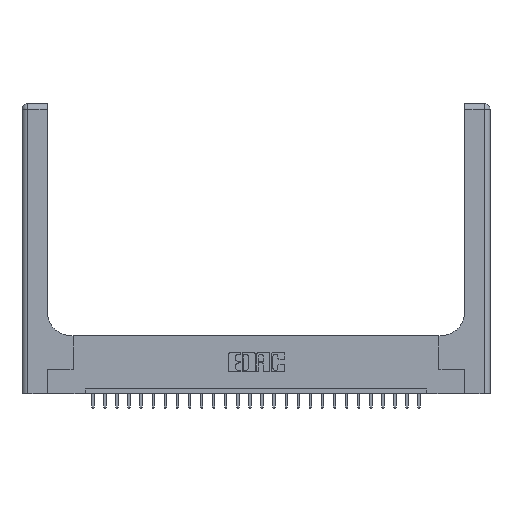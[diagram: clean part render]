
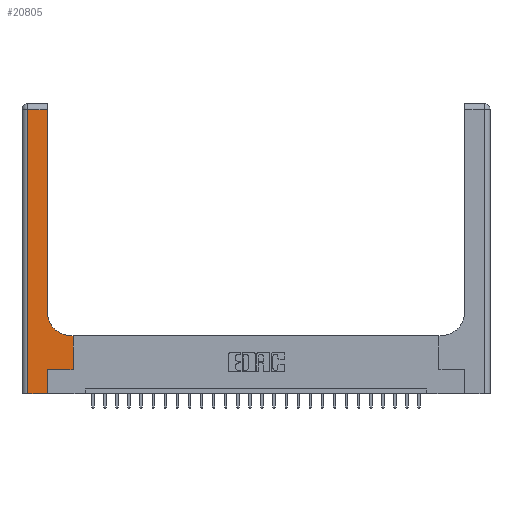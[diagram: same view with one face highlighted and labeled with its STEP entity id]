
A CAD part, top view. The second image highlights one B-rep face of the part: STEP entity #20805.
In plain terms, the highlighted planar face has unit normal (0, 0, 1).
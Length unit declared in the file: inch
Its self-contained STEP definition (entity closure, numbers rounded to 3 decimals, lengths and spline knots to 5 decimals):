
#198 = VERTEX_POINT ( 'NONE', #9054 ) ;
#216 = EDGE_CURVE ( 'NONE', #22967, #11953, #3012, .T. ) ;
#431 = CARTESIAN_POINT ( 'NONE',  ( 0.51, 0.6, 0.37 ) ) ;
#540 = ORIENTED_EDGE ( 'NONE', *, *, #24052, .T. ) ;
#685 = LINE ( 'NONE', #8869, #21875 ) ;
#1987 = CARTESIAN_POINT ( 'NONE',  ( 0.265, 0.25, 0.37 ) ) ;
#2176 = VERTEX_POINT ( 'NONE', #15925 ) ;
#2447 = DIRECTION ( 'NONE',  ( 0., 1., 0. ) ) ;
#2916 = DIRECTION ( 'NONE',  ( 1., 0., 0. ) ) ;
#3012 = LINE ( 'NONE', #6914, #24234 ) ;
#3833 = EDGE_CURVE ( 'NONE', #198, #21605, #20559, .T. ) ;
#4216 = CARTESIAN_POINT ( 'NONE',  ( 0.265, 0., 0.37 ) ) ;
#4338 = LINE ( 'NONE', #15784, #7513 ) ;
#4696 = AXIS2_PLACEMENT_3D ( 'NONE', #9134, #7483, #15160 ) ;
#4815 = CARTESIAN_POINT ( 'NONE',  ( 0.265, 0.25, 0.37 ) ) ;
#4822 = CARTESIAN_POINT ( 'NONE',  ( 0.26, 2.94, 0.37 ) ) ;
#5190 = CARTESIAN_POINT ( 'NONE',  ( 0.528, 0.6, 0.37 ) ) ;
#6422 = FACE_OUTER_BOUND ( 'NONE', #23594, .T. ) ;
#6914 = CARTESIAN_POINT ( 'NONE',  ( 0., 0., 0.37 ) ) ;
#7169 = DIRECTION ( 'NONE',  ( 1., 0., 0. ) ) ;
#7482 = DIRECTION ( 'NONE',  ( 0., 1., 0. ) ) ;
#7483 = DIRECTION ( 'NONE',  ( 0., 0., -1. ) ) ;
#7513 = VECTOR ( 'NONE', #2447, 39.37008 ) ;
#7598 = ORIENTED_EDGE ( 'NONE', *, *, #15189, .T. ) ;
#8093 = EDGE_CURVE ( 'NONE', #2176, #8866, #4338, .T. ) ;
#8492 = DIRECTION ( 'NONE',  ( 0., -1., 0. ) ) ;
#8735 = EDGE_CURVE ( 'NONE', #21010, #2176, #10728, .T. ) ;
#8866 = VERTEX_POINT ( 'NONE', #5190 ) ;
#8869 = CARTESIAN_POINT ( 'NONE',  ( 0.06, 3., 0.37 ) ) ;
#9054 = CARTESIAN_POINT ( 'NONE',  ( 0.26, 0.85, 0.37 ) ) ;
#9134 = CARTESIAN_POINT ( 'NONE',  ( 0.51, 0.85, 0.37 ) ) ;
#9492 = LINE ( 'NONE', #17180, #14533 ) ;
#9566 = EDGE_CURVE ( 'NONE', #21605, #9743, #12638, .T. ) ;
#9743 = VERTEX_POINT ( 'NONE', #17163 ) ;
#10199 = DIRECTION ( 'NONE',  ( 0., 0., -1. ) ) ;
#10326 = PLANE ( 'NONE',  #18311 ) ;
#10357 = DIRECTION ( 'NONE',  ( -1., 0., 0. ) ) ;
#10728 = LINE ( 'NONE', #4815, #22817 ) ;
#10981 = CARTESIAN_POINT ( 'NONE',  ( 0.26, 3., 0.37 ) ) ;
#11592 = VECTOR ( 'NONE', #15825, 39.37008 ) ;
#11953 = VERTEX_POINT ( 'NONE', #4216 ) ;
#12208 = DIRECTION ( 'NONE',  ( -1., 0., 0. ) ) ;
#12422 = ORIENTED_EDGE ( 'NONE', *, *, #3833, .T. ) ;
#12638 = LINE ( 'NONE', #19612, #11592 ) ;
#14093 = CARTESIAN_POINT ( 'NONE',  ( 0., 3., 0.37 ) ) ;
#14533 = VECTOR ( 'NONE', #7482, 39.37008 ) ;
#15160 = DIRECTION ( 'NONE',  ( 1., 0., 0. ) ) ;
#15189 = EDGE_CURVE ( 'NONE', #11953, #21010, #9492, .T. ) ;
#15447 = VECTOR ( 'NONE', #18679, 39.37008 ) ;
#15757 = ORIENTED_EDGE ( 'NONE', *, *, #8735, .T. ) ;
#15784 = CARTESIAN_POINT ( 'NONE',  ( 0.528, 0.25, 0.37 ) ) ;
#15825 = DIRECTION ( 'NONE',  ( -1., 0., 0. ) ) ;
#15925 = CARTESIAN_POINT ( 'NONE',  ( 0.528, 0.25, 0.37 ) ) ;
#16265 = VECTOR ( 'NONE', #10357, 39.37008 ) ;
#16843 = ORIENTED_EDGE ( 'NONE', *, *, #8093, .T. ) ;
#17163 = CARTESIAN_POINT ( 'NONE',  ( 0.06, 2.94, 0.37 ) ) ;
#17180 = CARTESIAN_POINT ( 'NONE',  ( 0.265, 0., 0.37 ) ) ;
#17415 = CARTESIAN_POINT ( 'NONE',  ( 0.06, 0., 0.37 ) ) ;
#18168 = CARTESIAN_POINT ( 'NONE',  ( 0.26, 0.6, 0.37 ) ) ;
#18311 = AXIS2_PLACEMENT_3D ( 'NONE', #14093, #10199, #12208 ) ;
#18679 = DIRECTION ( 'NONE',  ( 0., 1., 0. ) ) ;
#18900 = VERTEX_POINT ( 'NONE', #431 ) ;
#19612 = CARTESIAN_POINT ( 'NONE',  ( 0., 2.94, 0.37 ) ) ;
#19806 = EDGE_CURVE ( 'NONE', #9743, #22967, #685, .T. ) ;
#20326 = EDGE_CURVE ( 'NONE', #8866, #18900, #21814, .T. ) ;
#20559 = LINE ( 'NONE', #10981, #15447 ) ;
#20805 = ADVANCED_FACE ( 'NONE', ( #6422 ), #10326, .F. ) ;
#21010 = VERTEX_POINT ( 'NONE', #1987 ) ;
#21207 = ORIENTED_EDGE ( 'NONE', *, *, #216, .T. ) ;
#21455 = ORIENTED_EDGE ( 'NONE', *, *, #9566, .T. ) ;
#21605 = VERTEX_POINT ( 'NONE', #4822 ) ;
#21691 = ORIENTED_EDGE ( 'NONE', *, *, #20326, .T. ) ;
#21814 = LINE ( 'NONE', #18168, #16265 ) ;
#21875 = VECTOR ( 'NONE', #8492, 39.37008 ) ;
#22305 = ORIENTED_EDGE ( 'NONE', *, *, #19806, .T. ) ;
#22817 = VECTOR ( 'NONE', #2916, 39.37008 ) ;
#22967 = VERTEX_POINT ( 'NONE', #17415 ) ;
#23182 = CIRCLE ( 'NONE', #4696, 0.25 ) ;
#23594 = EDGE_LOOP ( 'NONE', ( #12422, #21455, #22305, #21207, #7598, #15757, #16843, #21691, #540 ) ) ;
#24052 = EDGE_CURVE ( 'NONE', #18900, #198, #23182, .T. ) ;
#24234 = VECTOR ( 'NONE', #7169, 39.37008 ) ;
